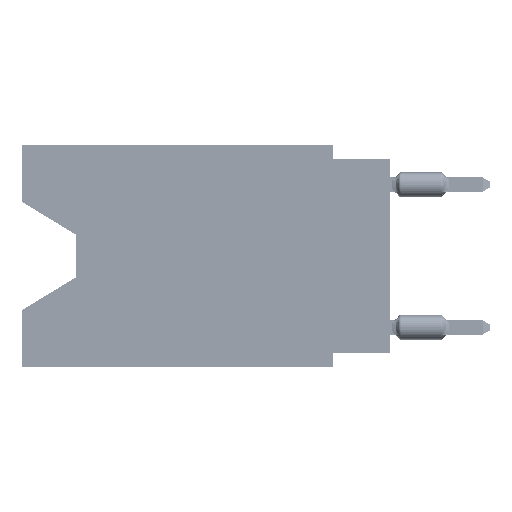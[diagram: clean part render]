
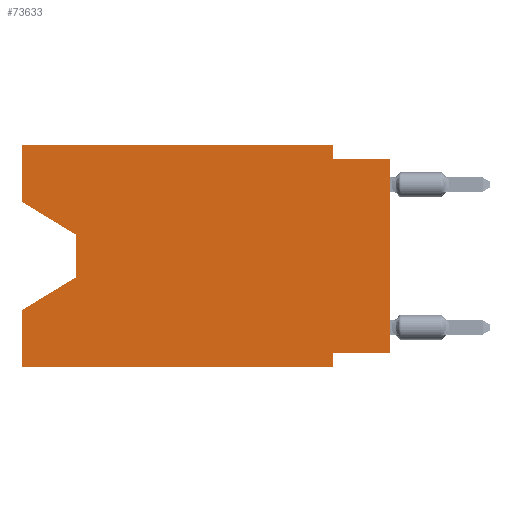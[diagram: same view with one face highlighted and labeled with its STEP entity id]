
A CAD part, left-side view. The second image highlights one B-rep face of the part: STEP entity #73633.
In plain terms, the highlighted planar face has unit normal (-1, 0, 0).
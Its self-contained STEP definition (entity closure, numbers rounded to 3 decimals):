
#311 = VERTEX_POINT ( 'NONE', #40732 ) ;
#497 = VECTOR ( 'NONE', #37687, 1000. ) ;
#1132 = AXIS2_PLACEMENT_3D ( 'NONE', #41652, #54038, #61297 ) ;
#1151 = CARTESIAN_POINT ( 'NONE',  ( 0., 16.383, -9.906 ) ) ;
#2616 = CARTESIAN_POINT ( 'NONE',  ( 0., 16.383, -2.546 ) ) ;
#2865 = EDGE_CURVE ( 'NONE', #48178, #311, #31358, .T. ) ;
#3749 = CARTESIAN_POINT ( 'NONE',  ( 0., 13.97, -5.893 ) ) ;
#4258 = ORIENTED_EDGE ( 'NONE', *, *, #50788, .F. ) ;
#5607 = DIRECTION ( 'NONE',  ( 0., -1., 0. ) ) ;
#6153 = ORIENTED_EDGE ( 'NONE', *, *, #76816, .F. ) ;
#7463 = ORIENTED_EDGE ( 'NONE', *, *, #12626, .F. ) ;
#7759 = EDGE_CURVE ( 'NONE', #26553, #57436, #52602, .T. ) ;
#8613 = VECTOR ( 'NONE', #17659, 1000. ) ;
#8993 = VERTEX_POINT ( 'NONE', #64767 ) ;
#9209 = PLANE ( 'NONE',  #1132 ) ;
#10350 = LINE ( 'NONE', #64138, #57774 ) ;
#11061 = DIRECTION ( 'NONE',  ( 0., 0., -1. ) ) ;
#11681 = VECTOR ( 'NONE', #37191, 1000. ) ;
#12626 = EDGE_CURVE ( 'NONE', #311, #77107, #81039, .T. ) ;
#12771 = LINE ( 'NONE', #52467, #55478 ) ;
#16671 = VECTOR ( 'NONE', #65330, 1000. ) ;
#17551 = LINE ( 'NONE', #23966, #11681 ) ;
#17659 = DIRECTION ( 'NONE',  ( 0., 0., -1. ) ) ;
#18061 = DIRECTION ( 'NONE',  ( 0., 0., 1. ) ) ;
#18316 = LINE ( 'NONE', #83273, #75574 ) ;
#19062 = EDGE_CURVE ( 'NONE', #31165, #57436, #69167, .T. ) ;
#20660 = CARTESIAN_POINT ( 'NONE',  ( 0., 0., -9.271 ) ) ;
#21844 = LINE ( 'NONE', #2616, #77975 ) ;
#22369 = ORIENTED_EDGE ( 'NONE', *, *, #2865, .F. ) ;
#23277 = CARTESIAN_POINT ( 'NONE',  ( 0., 16.383, 0. ) ) ;
#23718 = VERTEX_POINT ( 'NONE', #27338 ) ;
#23966 = CARTESIAN_POINT ( 'NONE',  ( 0., 0., -9.271 ) ) ;
#26553 = VERTEX_POINT ( 'NONE', #1151 ) ;
#26771 = ORIENTED_EDGE ( 'NONE', *, *, #46650, .T. ) ;
#26890 = LINE ( 'NONE', #76609, #8613 ) ;
#27217 = EDGE_CURVE ( 'NONE', #77107, #8993, #26890, .T. ) ;
#27338 = CARTESIAN_POINT ( 'NONE',  ( 0., 16.383, -7.36 ) ) ;
#29316 = DIRECTION ( 'NONE',  ( 0., -1., 0. ) ) ;
#30706 = DIRECTION ( 'NONE',  ( 0., 0.855, -0.519 ) ) ;
#31165 = VERTEX_POINT ( 'NONE', #52435 ) ;
#31358 = LINE ( 'NONE', #23277, #35507 ) ;
#32542 = LINE ( 'NONE', #76590, #38308 ) ;
#32958 = ORIENTED_EDGE ( 'NONE', *, *, #44846, .T. ) ;
#34669 = CARTESIAN_POINT ( 'NONE',  ( 0., 16.383, -2.546 ) ) ;
#35507 = VECTOR ( 'NONE', #62986, 1000. ) ;
#35585 = EDGE_LOOP ( 'NONE', ( #71433, #55131, #26771, #6153, #39036, #48804, #4258, #32958, #78022, #83505, #7463, #22369 ) ) ;
#37191 = DIRECTION ( 'NONE',  ( 0., 1., 0. ) ) ;
#37360 = VECTOR ( 'NONE', #29316, 1000. ) ;
#37687 = DIRECTION ( 'NONE',  ( 0., -1., 0. ) ) ;
#38308 = VECTOR ( 'NONE', #18061, 1000. ) ;
#39036 = ORIENTED_EDGE ( 'NONE', *, *, #7759, .T. ) ;
#40732 = CARTESIAN_POINT ( 'NONE',  ( 0., 16.383, 0. ) ) ;
#41652 = CARTESIAN_POINT ( 'NONE',  ( 0., 16.383, 0. ) ) ;
#43554 = VERTEX_POINT ( 'NONE', #3749 ) ;
#44101 = CARTESIAN_POINT ( 'NONE',  ( 0., 16.383, -9.906 ) ) ;
#44846 = EDGE_CURVE ( 'NONE', #75082, #57422, #66173, .T. ) ;
#46279 = EDGE_CURVE ( 'NONE', #8993, #57422, #10350, .T. ) ;
#46650 = EDGE_CURVE ( 'NONE', #43554, #23718, #18316, .T. ) ;
#47885 = DIRECTION ( 'NONE',  ( 0., -0.855, -0.519 ) ) ;
#48178 = VERTEX_POINT ( 'NONE', #34669 ) ;
#48804 = ORIENTED_EDGE ( 'NONE', *, *, #19062, .F. ) ;
#50788 = EDGE_CURVE ( 'NONE', #75082, #31165, #17551, .T. ) ;
#52435 = CARTESIAN_POINT ( 'NONE',  ( 0., 2.54, -9.271 ) ) ;
#52467 = CARTESIAN_POINT ( 'NONE',  ( 0., 13.97, -4.013 ) ) ;
#52602 = LINE ( 'NONE', #44101, #497 ) ;
#54038 = DIRECTION ( 'NONE',  ( 1., 0., 0. ) ) ;
#55131 = ORIENTED_EDGE ( 'NONE', *, *, #71565, .T. ) ;
#55478 = VECTOR ( 'NONE', #59300, 1000. ) ;
#57422 = VERTEX_POINT ( 'NONE', #65672 ) ;
#57436 = VERTEX_POINT ( 'NONE', #79752 ) ;
#57774 = VECTOR ( 'NONE', #5607, 1000. ) ;
#59300 = DIRECTION ( 'NONE',  ( 0., 0., -1. ) ) ;
#60151 = CARTESIAN_POINT ( 'NONE',  ( 0., 0., 0. ) ) ;
#61297 = DIRECTION ( 'NONE',  ( 0., 0., -1. ) ) ;
#62384 = CARTESIAN_POINT ( 'NONE',  ( 0., 2.54, 0. ) ) ;
#62986 = DIRECTION ( 'NONE',  ( 0., 0., 1. ) ) ;
#64138 = CARTESIAN_POINT ( 'NONE',  ( 0., 0., -0.635 ) ) ;
#64767 = CARTESIAN_POINT ( 'NONE',  ( 0., 2.54, -0.635 ) ) ;
#65330 = DIRECTION ( 'NONE',  ( 0., 0., 1. ) ) ;
#65672 = CARTESIAN_POINT ( 'NONE',  ( 0., 0., -0.635 ) ) ;
#66173 = LINE ( 'NONE', #60151, #16671 ) ;
#68752 = CARTESIAN_POINT ( 'NONE',  ( 0., 2.54, -9.906 ) ) ;
#69167 = LINE ( 'NONE', #68752, #83078 ) ;
#69946 = VERTEX_POINT ( 'NONE', #73067 ) ;
#71433 = ORIENTED_EDGE ( 'NONE', *, *, #82304, .T. ) ;
#71565 = EDGE_CURVE ( 'NONE', #69946, #43554, #12771, .T. ) ;
#73067 = CARTESIAN_POINT ( 'NONE',  ( 0., 13.97, -4.013 ) ) ;
#73633 = ADVANCED_FACE ( 'NONE', ( #74974 ), #9209, .F. ) ;
#74616 = CARTESIAN_POINT ( 'NONE',  ( 0., 16.383, 0. ) ) ;
#74974 = FACE_OUTER_BOUND ( 'NONE', #35585, .T. ) ;
#75082 = VERTEX_POINT ( 'NONE', #20660 ) ;
#75574 = VECTOR ( 'NONE', #30706, 1000. ) ;
#76590 = CARTESIAN_POINT ( 'NONE',  ( 0., 16.383, 0. ) ) ;
#76609 = CARTESIAN_POINT ( 'NONE',  ( 0., 2.54, 0. ) ) ;
#76816 = EDGE_CURVE ( 'NONE', #26553, #23718, #32542, .T. ) ;
#77107 = VERTEX_POINT ( 'NONE', #62384 ) ;
#77975 = VECTOR ( 'NONE', #47885, 1000. ) ;
#78022 = ORIENTED_EDGE ( 'NONE', *, *, #46279, .F. ) ;
#79752 = CARTESIAN_POINT ( 'NONE',  ( 0., 2.54, -9.906 ) ) ;
#81039 = LINE ( 'NONE', #74616, #37360 ) ;
#82304 = EDGE_CURVE ( 'NONE', #48178, #69946, #21844, .T. ) ;
#83078 = VECTOR ( 'NONE', #11061, 1000. ) ;
#83273 = CARTESIAN_POINT ( 'NONE',  ( 0., 13.97, -5.893 ) ) ;
#83505 = ORIENTED_EDGE ( 'NONE', *, *, #27217, .F. ) ;
